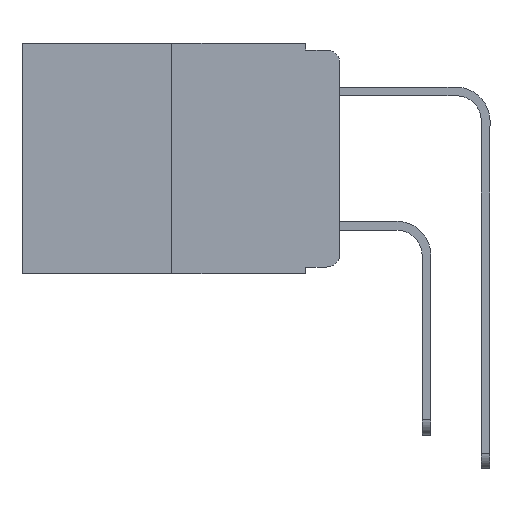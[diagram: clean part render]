
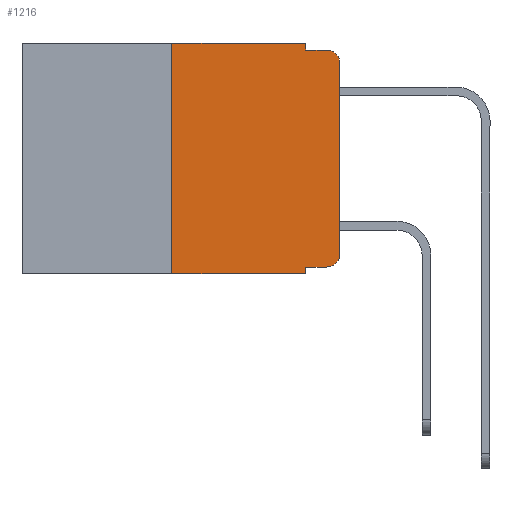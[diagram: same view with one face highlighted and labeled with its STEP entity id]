
A CAD part, left-side view. The second image highlights one B-rep face of the part: STEP entity #1216.
In plain terms, the highlighted planar face has unit normal (-1, 0, 0).
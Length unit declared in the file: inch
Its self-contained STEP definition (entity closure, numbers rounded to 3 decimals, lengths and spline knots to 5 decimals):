
#20 = VECTOR ( 'NONE', #4285, 39.37008 ) ;
#37 = EDGE_CURVE ( 'NONE', #3749, #2332, #1589, .T. ) ;
#52 = CIRCLE ( 'NONE', #160, 0.02 ) ;
#93 = CARTESIAN_POINT ( 'NONE',  ( 0., 0.25, 0. ) ) ;
#160 = AXIS2_PLACEMENT_3D ( 'NONE', #12923, #12953, #4219 ) ;
#168 = LINE ( 'NONE', #2245, #7723 ) ;
#493 = DIRECTION ( 'NONE',  ( 1., 0., 0. ) ) ;
#744 = CARTESIAN_POINT ( 'NONE',  ( 0., 0., -0.03 ) ) ;
#1010 = ORIENTED_EDGE ( 'NONE', *, *, #2454, .T. ) ;
#1216 = ADVANCED_FACE ( 'NONE', ( #9204 ), #3535, .F. ) ;
#1523 = EDGE_CURVE ( 'NONE', #8262, #4839, #7769, .T. ) ;
#1575 = CARTESIAN_POINT ( 'NONE',  ( 0., 0., -0.313 ) ) ;
#1589 = LINE ( 'NONE', #4075, #9380 ) ;
#1592 = CARTESIAN_POINT ( 'NONE',  ( 0., 0.051, -0.333 ) ) ;
#1676 = ORIENTED_EDGE ( 'NONE', *, *, #8909, .F. ) ;
#1709 = VECTOR ( 'NONE', #3909, 39.37008 ) ;
#2107 = CARTESIAN_POINT ( 'NONE',  ( 0., 0.051, -0.333 ) ) ;
#2138 = LINE ( 'NONE', #2107, #9918 ) ;
#2148 = DIRECTION ( 'NONE',  ( 0., -1., 0. ) ) ;
#2190 = DIRECTION ( 'NONE',  ( 0., 0., 1. ) ) ;
#2240 = CARTESIAN_POINT ( 'NONE',  ( 0., 0.473, 0. ) ) ;
#2245 = CARTESIAN_POINT ( 'NONE',  ( 0., 0.473, -0.343 ) ) ;
#2332 = VERTEX_POINT ( 'NONE', #3303 ) ;
#2341 = EDGE_CURVE ( 'NONE', #8000, #12441, #4149, .T. ) ;
#2384 = CARTESIAN_POINT ( 'NONE',  ( 0., 0.02, -0.313 ) ) ;
#2454 = EDGE_CURVE ( 'NONE', #11156, #2332, #52, .T. ) ;
#2858 = DIRECTION ( 'NONE',  ( 0., -1., 0. ) ) ;
#3029 = EDGE_LOOP ( 'NONE', ( #10870, #1010, #8540, #1676, #4108, #10088, #12396, #10723, #10389, #8705 ) ) ;
#3303 = CARTESIAN_POINT ( 'NONE',  ( 0., 0.02, -0.01 ) ) ;
#3431 = DIRECTION ( 'NONE',  ( 0., 0., -1. ) ) ;
#3535 = PLANE ( 'NONE',  #12963 ) ;
#3749 = VERTEX_POINT ( 'NONE', #9902 ) ;
#3812 = EDGE_CURVE ( 'NONE', #10347, #11156, #5518, .T. ) ;
#3909 = DIRECTION ( 'NONE',  ( 0., 0., -1. ) ) ;
#4029 = EDGE_CURVE ( 'NONE', #10922, #12441, #168, .T. ) ;
#4075 = CARTESIAN_POINT ( 'NONE',  ( 0., 0.051, -0.01 ) ) ;
#4108 = ORIENTED_EDGE ( 'NONE', *, *, #1523, .F. ) ;
#4149 = LINE ( 'NONE', #10414, #1709 ) ;
#4219 = DIRECTION ( 'NONE',  ( 0., 0., -1. ) ) ;
#4255 = CARTESIAN_POINT ( 'NONE',  ( 0., 0., 0. ) ) ;
#4285 = DIRECTION ( 'NONE',  ( 0., 0., 1. ) ) ;
#4538 = LINE ( 'NONE', #93, #6859 ) ;
#4585 = CIRCLE ( 'NONE', #5658, 0.02 ) ;
#4839 = VERTEX_POINT ( 'NONE', #5786 ) ;
#5108 = CARTESIAN_POINT ( 'NONE',  ( 0., 0.25, 0. ) ) ;
#5398 = VECTOR ( 'NONE', #2858, 39.37008 ) ;
#5518 = LINE ( 'NONE', #4255, #20 ) ;
#5647 = CARTESIAN_POINT ( 'NONE',  ( 0., 0.02, -0.333 ) ) ;
#5658 = AXIS2_PLACEMENT_3D ( 'NONE', #2384, #9486, #3431 ) ;
#5786 = CARTESIAN_POINT ( 'NONE',  ( 0., 0.051, 0. ) ) ;
#6292 = VERTEX_POINT ( 'NONE', #5647 ) ;
#6764 = CARTESIAN_POINT ( 'NONE',  ( 0., 0.473, 0. ) ) ;
#6859 = VECTOR ( 'NONE', #2190, 39.37008 ) ;
#7510 = CARTESIAN_POINT ( 'NONE',  ( 0., 0.25, -0.343 ) ) ;
#7723 = VECTOR ( 'NONE', #2148, 39.37008 ) ;
#7769 = LINE ( 'NONE', #6764, #5398 ) ;
#8000 = VERTEX_POINT ( 'NONE', #1592 ) ;
#8165 = CARTESIAN_POINT ( 'NONE',  ( 0., 0.051, 0. ) ) ;
#8262 = VERTEX_POINT ( 'NONE', #5108 ) ;
#8505 = EDGE_CURVE ( 'NONE', #6292, #10347, #4585, .T. ) ;
#8540 = ORIENTED_EDGE ( 'NONE', *, *, #37, .F. ) ;
#8705 = ORIENTED_EDGE ( 'NONE', *, *, #8505, .T. ) ;
#8909 = EDGE_CURVE ( 'NONE', #4839, #3749, #10860, .T. ) ;
#8926 = EDGE_CURVE ( 'NONE', #8000, #6292, #2138, .T. ) ;
#9204 = FACE_OUTER_BOUND ( 'NONE', #3029, .T. ) ;
#9380 = VECTOR ( 'NONE', #11857, 39.37008 ) ;
#9486 = DIRECTION ( 'NONE',  ( -1., 0., 0. ) ) ;
#9902 = CARTESIAN_POINT ( 'NONE',  ( 0., 0.051, -0.01 ) ) ;
#9918 = VECTOR ( 'NONE', #10223, 39.37008 ) ;
#10088 = ORIENTED_EDGE ( 'NONE', *, *, #11898, .F. ) ;
#10223 = DIRECTION ( 'NONE',  ( 0., -1., 0. ) ) ;
#10347 = VERTEX_POINT ( 'NONE', #1575 ) ;
#10389 = ORIENTED_EDGE ( 'NONE', *, *, #8926, .T. ) ;
#10414 = CARTESIAN_POINT ( 'NONE',  ( 0., 0.051, 0. ) ) ;
#10541 = VECTOR ( 'NONE', #12107, 39.37008 ) ;
#10723 = ORIENTED_EDGE ( 'NONE', *, *, #2341, .F. ) ;
#10860 = LINE ( 'NONE', #8165, #10541 ) ;
#10870 = ORIENTED_EDGE ( 'NONE', *, *, #3812, .T. ) ;
#10879 = DIRECTION ( 'NONE',  ( 0., 0., -1. ) ) ;
#10922 = VERTEX_POINT ( 'NONE', #7510 ) ;
#11156 = VERTEX_POINT ( 'NONE', #744 ) ;
#11857 = DIRECTION ( 'NONE',  ( 0., -1., 0. ) ) ;
#11898 = EDGE_CURVE ( 'NONE', #10922, #8262, #4538, .T. ) ;
#12107 = DIRECTION ( 'NONE',  ( 0., 0., -1. ) ) ;
#12140 = CARTESIAN_POINT ( 'NONE',  ( 0., 0.051, -0.343 ) ) ;
#12396 = ORIENTED_EDGE ( 'NONE', *, *, #4029, .T. ) ;
#12441 = VERTEX_POINT ( 'NONE', #12140 ) ;
#12923 = CARTESIAN_POINT ( 'NONE',  ( 0., 0.02, -0.03 ) ) ;
#12953 = DIRECTION ( 'NONE',  ( -1., 0., 0. ) ) ;
#12963 = AXIS2_PLACEMENT_3D ( 'NONE', #2240, #493, #10879 ) ;
